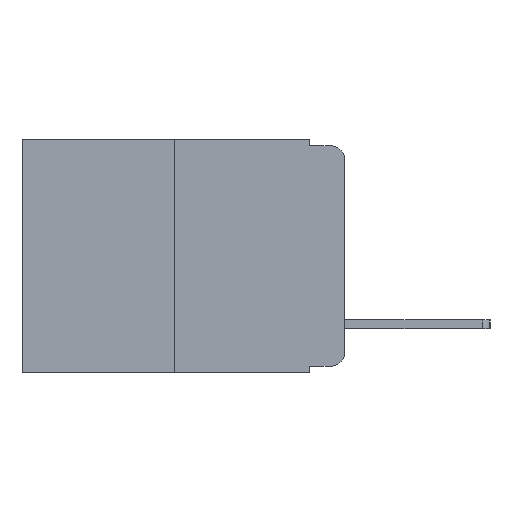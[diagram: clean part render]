
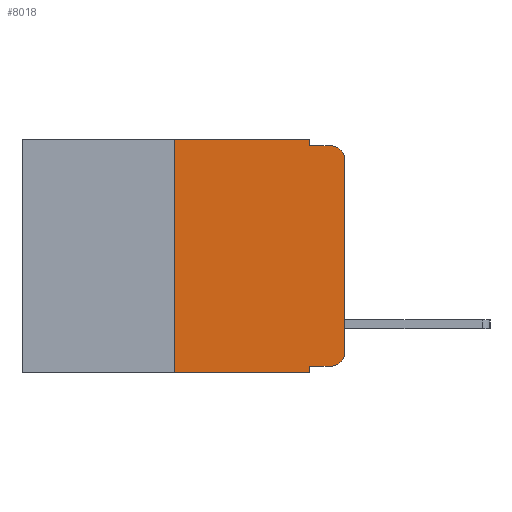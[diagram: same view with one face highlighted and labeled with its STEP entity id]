
A CAD part, left-side view. The second image highlights one B-rep face of the part: STEP entity #8018.
In plain terms, the highlighted planar face has unit normal (-1, 0, 0).
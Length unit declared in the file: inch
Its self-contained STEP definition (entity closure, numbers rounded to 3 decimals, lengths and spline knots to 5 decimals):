
#89 = VERTEX_POINT ( 'NONE', #9767 ) ;
#90 = AXIS2_PLACEMENT_3D ( 'NONE', #9930, #8176, #2109 ) ;
#166 = CARTESIAN_POINT ( 'NONE',  ( 0., 0.051, 0. ) ) ;
#436 = DIRECTION ( 'NONE',  ( 0., -1., 0. ) ) ;
#699 = CARTESIAN_POINT ( 'NONE',  ( 0., 0.25, 0. ) ) ;
#1070 = PLANE ( 'NONE',  #90 ) ;
#1364 = CARTESIAN_POINT ( 'NONE',  ( 0., 0.051, -0.01 ) ) ;
#1687 = ORIENTED_EDGE ( 'NONE', *, *, #7032, .F. ) ;
#1964 = FACE_OUTER_BOUND ( 'NONE', #8084, .T. ) ;
#2109 = DIRECTION ( 'NONE',  ( 0., 0., -1. ) ) ;
#2169 = VECTOR ( 'NONE', #11877, 39.37008 ) ;
#2282 = VERTEX_POINT ( 'NONE', #4946 ) ;
#2291 = CARTESIAN_POINT ( 'NONE',  ( 0., 0.051, -0.01 ) ) ;
#2327 = VECTOR ( 'NONE', #9764, 39.37008 ) ;
#2457 = DIRECTION ( 'NONE',  ( 0., 0., 1. ) ) ;
#2498 = VECTOR ( 'NONE', #2457, 39.37008 ) ;
#2569 = AXIS2_PLACEMENT_3D ( 'NONE', #9474, #3593, #10312 ) ;
#2832 = LINE ( 'NONE', #1364, #4668 ) ;
#3149 = CIRCLE ( 'NONE', #12143, 0.02 ) ;
#3418 = CARTESIAN_POINT ( 'NONE',  ( 0., 0., 0. ) ) ;
#3480 = ORIENTED_EDGE ( 'NONE', *, *, #6995, .T. ) ;
#3593 = DIRECTION ( 'NONE',  ( -1., 0., 0. ) ) ;
#3893 = LINE ( 'NONE', #11570, #5915 ) ;
#4500 = CARTESIAN_POINT ( 'NONE',  ( 0., 0.02, -0.03 ) ) ;
#4668 = VECTOR ( 'NONE', #7487, 39.37008 ) ;
#4912 = CARTESIAN_POINT ( 'NONE',  ( 0., 0.051, -0.333 ) ) ;
#4946 = CARTESIAN_POINT ( 'NONE',  ( 0., 0.02, -0.333 ) ) ;
#5116 = EDGE_CURVE ( 'NONE', #8791, #10684, #3893, .T. ) ;
#5504 = DIRECTION ( 'NONE',  ( 0., 0., -1. ) ) ;
#5546 = VECTOR ( 'NONE', #8430, 39.37008 ) ;
#5593 = CARTESIAN_POINT ( 'NONE',  ( 0., 0.051, 0. ) ) ;
#5915 = VECTOR ( 'NONE', #7201, 39.37008 ) ;
#6141 = ORIENTED_EDGE ( 'NONE', *, *, #6999, .F. ) ;
#6142 = VECTOR ( 'NONE', #8472, 39.37008 ) ;
#6224 = VERTEX_POINT ( 'NONE', #11545 ) ;
#6445 = ORIENTED_EDGE ( 'NONE', *, *, #5116, .F. ) ;
#6475 = CARTESIAN_POINT ( 'NONE',  ( 0., 0.25, 0. ) ) ;
#6745 = EDGE_CURVE ( 'NONE', #11449, #7338, #11753, .T. ) ;
#6781 = ORIENTED_EDGE ( 'NONE', *, *, #6745, .T. ) ;
#6993 = EDGE_CURVE ( 'NONE', #89, #6224, #8189, .T. ) ;
#6995 = EDGE_CURVE ( 'NONE', #6224, #11076, #3149, .T. ) ;
#6999 = EDGE_CURVE ( 'NONE', #10723, #11076, #2832, .T. ) ;
#7016 = EDGE_CURVE ( 'NONE', #10684, #10723, #10525, .T. ) ;
#7019 = EDGE_CURVE ( 'NONE', #11449, #8791, #10258, .T. ) ;
#7032 = EDGE_CURVE ( 'NONE', #11438, #7338, #11875, .T. ) ;
#7037 = EDGE_CURVE ( 'NONE', #11438, #2282, #7905, .T. ) ;
#7040 = EDGE_CURVE ( 'NONE', #2282, #89, #9727, .T. ) ;
#7107 = ORIENTED_EDGE ( 'NONE', *, *, #7037, .T. ) ;
#7201 = DIRECTION ( 'NONE',  ( 0., -1., 0. ) ) ;
#7273 = VECTOR ( 'NONE', #436, 39.37008 ) ;
#7338 = VERTEX_POINT ( 'NONE', #9178 ) ;
#7487 = DIRECTION ( 'NONE',  ( 0., -1., 0. ) ) ;
#7532 = CARTESIAN_POINT ( 'NONE',  ( 0., 0.051, 0. ) ) ;
#7905 = LINE ( 'NONE', #10210, #7273 ) ;
#8018 = ADVANCED_FACE ( 'NONE', ( #1964 ), #1070, .F. ) ;
#8084 = EDGE_LOOP ( 'NONE', ( #8467, #3480, #6141, #11014, #6445, #11270, #6781, #1687, #7107, #9603 ) ) ;
#8176 = DIRECTION ( 'NONE',  ( 1., 0., 0. ) ) ;
#8189 = LINE ( 'NONE', #3418, #5546 ) ;
#8430 = DIRECTION ( 'NONE',  ( 0., 0., 1. ) ) ;
#8467 = ORIENTED_EDGE ( 'NONE', *, *, #6993, .T. ) ;
#8472 = DIRECTION ( 'NONE',  ( 0., 0., -1. ) ) ;
#8791 = VERTEX_POINT ( 'NONE', #699 ) ;
#8874 = CARTESIAN_POINT ( 'NONE',  ( 0., 0.473, -0.343 ) ) ;
#9178 = CARTESIAN_POINT ( 'NONE',  ( 0., 0.051, -0.343 ) ) ;
#9474 = CARTESIAN_POINT ( 'NONE',  ( 0., 0.02, -0.313 ) ) ;
#9603 = ORIENTED_EDGE ( 'NONE', *, *, #7040, .T. ) ;
#9727 = CIRCLE ( 'NONE', #2569, 0.02 ) ;
#9764 = DIRECTION ( 'NONE',  ( 0., -1., 0. ) ) ;
#9767 = CARTESIAN_POINT ( 'NONE',  ( 0., 0., -0.313 ) ) ;
#9930 = CARTESIAN_POINT ( 'NONE',  ( 0., 0.473, 0. ) ) ;
#10210 = CARTESIAN_POINT ( 'NONE',  ( 0., 0.051, -0.333 ) ) ;
#10258 = LINE ( 'NONE', #6475, #2498 ) ;
#10312 = DIRECTION ( 'NONE',  ( 0., 0., -1. ) ) ;
#10319 = CARTESIAN_POINT ( 'NONE',  ( 0., 0.02, -0.01 ) ) ;
#10525 = LINE ( 'NONE', #7532, #6142 ) ;
#10684 = VERTEX_POINT ( 'NONE', #166 ) ;
#10723 = VERTEX_POINT ( 'NONE', #2291 ) ;
#11014 = ORIENTED_EDGE ( 'NONE', *, *, #7016, .F. ) ;
#11018 = DIRECTION ( 'NONE',  ( -1., 0., 0. ) ) ;
#11076 = VERTEX_POINT ( 'NONE', #10319 ) ;
#11270 = ORIENTED_EDGE ( 'NONE', *, *, #7019, .F. ) ;
#11339 = CARTESIAN_POINT ( 'NONE',  ( 0., 0.25, -0.343 ) ) ;
#11438 = VERTEX_POINT ( 'NONE', #4912 ) ;
#11449 = VERTEX_POINT ( 'NONE', #11339 ) ;
#11545 = CARTESIAN_POINT ( 'NONE',  ( 0., 0., -0.03 ) ) ;
#11570 = CARTESIAN_POINT ( 'NONE',  ( 0., 0.473, 0. ) ) ;
#11753 = LINE ( 'NONE', #8874, #2327 ) ;
#11875 = LINE ( 'NONE', #5593, #2169 ) ;
#11877 = DIRECTION ( 'NONE',  ( 0., 0., -1. ) ) ;
#12143 = AXIS2_PLACEMENT_3D ( 'NONE', #4500, #11018, #5504 ) ;
